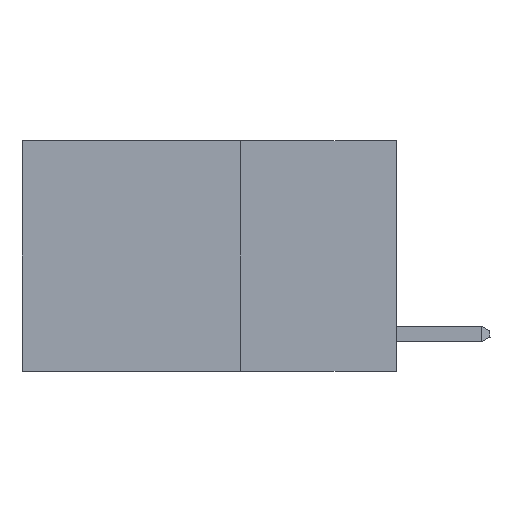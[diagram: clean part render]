
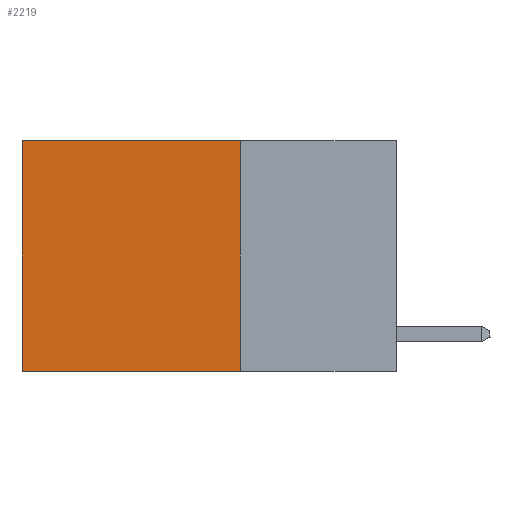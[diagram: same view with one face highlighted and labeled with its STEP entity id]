
A CAD part, left-side view. The second image highlights one B-rep face of the part: STEP entity #2219.
In plain terms, the highlighted planar face has unit normal (-1, 0, 0).
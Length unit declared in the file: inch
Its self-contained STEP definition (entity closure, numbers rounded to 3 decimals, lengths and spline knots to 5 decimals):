
#442 = VERTEX_POINT ( 'NONE', #2624 ) ;
#561 = VERTEX_POINT ( 'NONE', #1801 ) ;
#1737 = VERTEX_POINT ( 'NONE', #11210 ) ;
#1801 = CARTESIAN_POINT ( 'NONE',  ( 0.2625, 0.25, 0. ) ) ;
#1887 = LINE ( 'NONE', #11475, #6986 ) ;
#1890 = CARTESIAN_POINT ( 'NONE',  ( 0.2625, 0.25, 0. ) ) ;
#1968 = ORIENTED_EDGE ( 'NONE', *, *, #10528, .F. ) ;
#2070 = ORIENTED_EDGE ( 'NONE', *, *, #5353, .F. ) ;
#2197 = VECTOR ( 'NONE', #12048, 39.37008 ) ;
#2219 = ADVANCED_FACE ( 'NONE', ( #2937 ), #3791, .F. ) ;
#2240 = CARTESIAN_POINT ( 'NONE',  ( 0.2625, 0.25, -0.37 ) ) ;
#2624 = CARTESIAN_POINT ( 'NONE',  ( 0.2625, 0.25, -0.37 ) ) ;
#2937 = FACE_OUTER_BOUND ( 'NONE', #9370, .T. ) ;
#2982 = VERTEX_POINT ( 'NONE', #9079 ) ;
#3015 = ORIENTED_EDGE ( 'NONE', *, *, #6247, .T. ) ;
#3791 = PLANE ( 'NONE',  #12914 ) ;
#4669 = VECTOR ( 'NONE', #9332, 39.37008 ) ;
#4811 = DIRECTION ( 'NONE',  ( 1., 0., 0. ) ) ;
#5111 = LINE ( 'NONE', #2240, #12580 ) ;
#5310 = DIRECTION ( 'NONE',  ( 0., 1., 0. ) ) ;
#5353 = EDGE_CURVE ( 'NONE', #561, #442, #1887, .T. ) ;
#6247 = EDGE_CURVE ( 'NONE', #561, #1737, #10021, .T. ) ;
#6986 = VECTOR ( 'NONE', #8461, 39.37008 ) ;
#7314 = CARTESIAN_POINT ( 'NONE',  ( 0.2625, 0.6, 0. ) ) ;
#7794 = ORIENTED_EDGE ( 'NONE', *, *, #8985, .T. ) ;
#8461 = DIRECTION ( 'NONE',  ( 0., 0., -1. ) ) ;
#8985 = EDGE_CURVE ( 'NONE', #1737, #2982, #12471, .T. ) ;
#9079 = CARTESIAN_POINT ( 'NONE',  ( 0.2625, 0.6, -0.37 ) ) ;
#9332 = DIRECTION ( 'NONE',  ( 0., 0., -1. ) ) ;
#9370 = EDGE_LOOP ( 'NONE', ( #7794, #1968, #2070, #3015 ) ) ;
#10021 = LINE ( 'NONE', #1890, #2197 ) ;
#10528 = EDGE_CURVE ( 'NONE', #442, #2982, #5111, .T. ) ;
#10934 = CARTESIAN_POINT ( 'NONE',  ( 0.2625, 0.25, 0. ) ) ;
#11210 = CARTESIAN_POINT ( 'NONE',  ( 0.2625, 0.6, 0. ) ) ;
#11475 = CARTESIAN_POINT ( 'NONE',  ( 0.2625, 0.25, 0. ) ) ;
#11928 = DIRECTION ( 'NONE',  ( 0., 0., -1. ) ) ;
#12048 = DIRECTION ( 'NONE',  ( 0., 1., 0. ) ) ;
#12471 = LINE ( 'NONE', #7314, #4669 ) ;
#12580 = VECTOR ( 'NONE', #5310, 39.37008 ) ;
#12914 = AXIS2_PLACEMENT_3D ( 'NONE', #10934, #4811, #11928 ) ;
